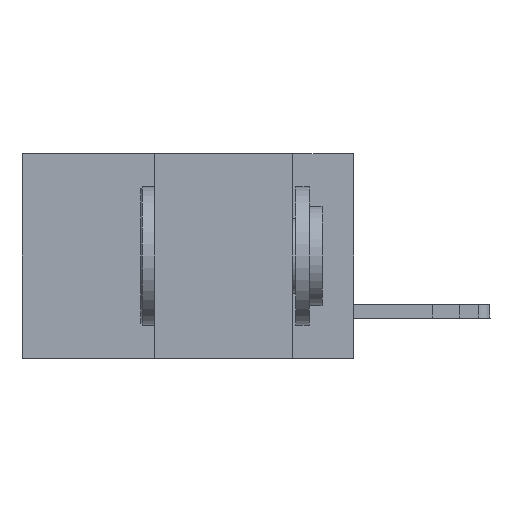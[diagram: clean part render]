
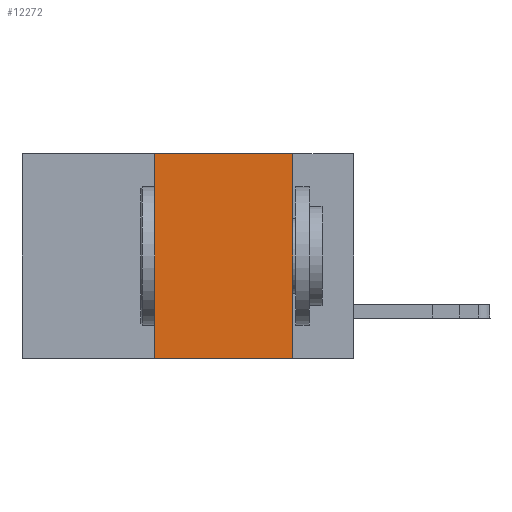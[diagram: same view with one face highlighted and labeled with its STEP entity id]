
A CAD part, left-side view. The second image highlights one B-rep face of the part: STEP entity #12272.
In plain terms, the highlighted planar face has unit normal (-1, 0, 0).
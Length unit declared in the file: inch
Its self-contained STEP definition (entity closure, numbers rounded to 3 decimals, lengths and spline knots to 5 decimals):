
#670 = EDGE_LOOP ( 'NONE', ( #7958, #17573, #3299, #16005 ) ) ;
#1951 = VECTOR ( 'NONE', #3691, 39.37008 ) ;
#2227 = EDGE_CURVE ( 'NONE', #13015, #11372, #8366, .T. ) ;
#3232 = VECTOR ( 'NONE', #31878, 39.37008 ) ;
#3299 = ORIENTED_EDGE ( 'NONE', *, *, #22531, .F. ) ;
#3691 = DIRECTION ( 'NONE',  ( 0., -1., 0. ) ) ;
#3849 = VERTEX_POINT ( 'NONE', #5498 ) ;
#4692 = DIRECTION ( 'NONE',  ( 0., 0., 1. ) ) ;
#5498 = CARTESIAN_POINT ( 'NONE',  ( 0., 0.11, 0. ) ) ;
#6351 = CARTESIAN_POINT ( 'NONE',  ( 0., 0.6, -0.37 ) ) ;
#7958 = ORIENTED_EDGE ( 'NONE', *, *, #23610, .F. ) ;
#8366 = LINE ( 'NONE', #6351, #3232 ) ;
#9690 = VECTOR ( 'NONE', #4692, 39.37008 ) ;
#11372 = VERTEX_POINT ( 'NONE', #26278 ) ;
#12272 = ADVANCED_FACE ( 'NONE', ( #18872 ), #19039, .F. ) ;
#13015 = VERTEX_POINT ( 'NONE', #18172 ) ;
#14866 = CARTESIAN_POINT ( 'NONE',  ( 0., 0.36, 0. ) ) ;
#16005 = ORIENTED_EDGE ( 'NONE', *, *, #2227, .T. ) ;
#16697 = EDGE_CURVE ( 'NONE', #26496, #3849, #19042, .T. ) ;
#16703 = CARTESIAN_POINT ( 'NONE',  ( 0., 0.6, 0. ) ) ;
#17573 = ORIENTED_EDGE ( 'NONE', *, *, #16697, .F. ) ;
#17632 = VECTOR ( 'NONE', #23115, 39.37008 ) ;
#17795 = CARTESIAN_POINT ( 'NONE',  ( 0., 0.11, 0. ) ) ;
#18172 = CARTESIAN_POINT ( 'NONE',  ( 0., 0.36, -0.37 ) ) ;
#18872 = FACE_OUTER_BOUND ( 'NONE', #670, .T. ) ;
#19039 = PLANE ( 'NONE',  #32066 ) ;
#19042 = LINE ( 'NONE', #16703, #1951 ) ;
#22516 = CARTESIAN_POINT ( 'NONE',  ( 0., 0.36, 0. ) ) ;
#22531 = EDGE_CURVE ( 'NONE', #13015, #26496, #27368, .T. ) ;
#23115 = DIRECTION ( 'NONE',  ( 0., 0., -1. ) ) ;
#23361 = DIRECTION ( 'NONE',  ( 0., 0., -1. ) ) ;
#23610 = EDGE_CURVE ( 'NONE', #3849, #11372, #28114, .T. ) ;
#23865 = DIRECTION ( 'NONE',  ( 1., 0., 0. ) ) ;
#26033 = CARTESIAN_POINT ( 'NONE',  ( 0., 0.6, 0. ) ) ;
#26278 = CARTESIAN_POINT ( 'NONE',  ( 0., 0.11, -0.37 ) ) ;
#26496 = VERTEX_POINT ( 'NONE', #22516 ) ;
#27368 = LINE ( 'NONE', #14866, #9690 ) ;
#28114 = LINE ( 'NONE', #17795, #17632 ) ;
#31878 = DIRECTION ( 'NONE',  ( 0., -1., 0. ) ) ;
#32066 = AXIS2_PLACEMENT_3D ( 'NONE', #26033, #23865, #23361 ) ;
